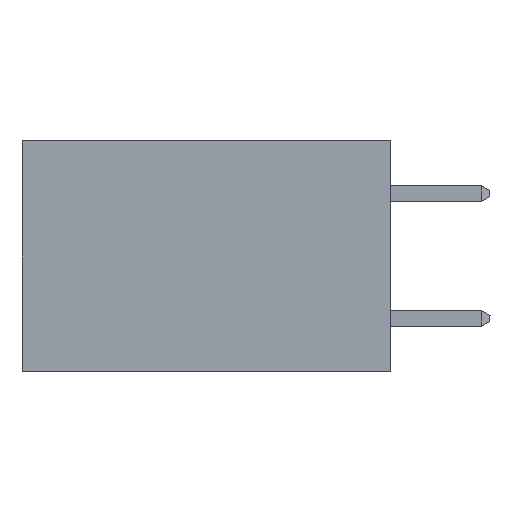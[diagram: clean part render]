
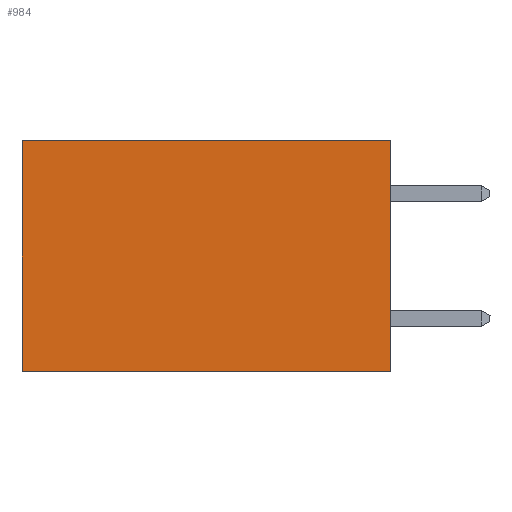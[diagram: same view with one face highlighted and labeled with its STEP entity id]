
A CAD part, left-side view. The second image highlights one B-rep face of the part: STEP entity #984.
In plain terms, the highlighted planar face has unit normal (-1, 0, 0).
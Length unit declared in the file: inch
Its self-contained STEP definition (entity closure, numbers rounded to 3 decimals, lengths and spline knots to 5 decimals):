
#61 = EDGE_CURVE ( 'NONE', #12855, #1841, #12094, .T. ) ;
#277 = DIRECTION ( 'NONE',  ( 0., 0., -1. ) ) ;
#730 = DIRECTION ( 'NONE',  ( 0., 1., 0. ) ) ;
#984 = ADVANCED_FACE ( 'NONE', ( #10764 ), #16046, .F. ) ;
#1525 = LINE ( 'NONE', #8451, #9704 ) ;
#1716 = ORIENTED_EDGE ( 'NONE', *, *, #5894, .F. ) ;
#1841 = VERTEX_POINT ( 'NONE', #11664 ) ;
#2413 = VECTOR ( 'NONE', #17200, 39.37008 ) ;
#2442 = DIRECTION ( 'NONE',  ( 1., 0., 0. ) ) ;
#2980 = ORIENTED_EDGE ( 'NONE', *, *, #6045, .F. ) ;
#4215 = CARTESIAN_POINT ( 'NONE',  ( 0.277, 0., 0. ) ) ;
#5894 = EDGE_CURVE ( 'NONE', #10501, #14128, #12106, .T. ) ;
#6045 = EDGE_CURVE ( 'NONE', #12855, #10501, #20850, .T. ) ;
#6291 = ORIENTED_EDGE ( 'NONE', *, *, #61, .T. ) ;
#6987 = EDGE_LOOP ( 'NONE', ( #19862, #1716, #2980, #6291 ) ) ;
#8206 = CARTESIAN_POINT ( 'NONE',  ( 0.277, 0., -0.37 ) ) ;
#8451 = CARTESIAN_POINT ( 'NONE',  ( 0.277, 0.59, -0.37 ) ) ;
#9471 = DIRECTION ( 'NONE',  ( 0., 0., -1. ) ) ;
#9704 = VECTOR ( 'NONE', #277, 39.37008 ) ;
#10501 = VERTEX_POINT ( 'NONE', #8206 ) ;
#10764 = FACE_OUTER_BOUND ( 'NONE', #6987, .T. ) ;
#11664 = CARTESIAN_POINT ( 'NONE',  ( 0.277, 0.59, 0. ) ) ;
#11853 = VECTOR ( 'NONE', #9471, 39.37008 ) ;
#12094 = LINE ( 'NONE', #4215, #20114 ) ;
#12106 = LINE ( 'NONE', #16774, #2413 ) ;
#12453 = CARTESIAN_POINT ( 'NONE',  ( 0.277, 0., -0.37 ) ) ;
#12855 = VERTEX_POINT ( 'NONE', #15340 ) ;
#14128 = VERTEX_POINT ( 'NONE', #15090 ) ;
#14478 = DIRECTION ( 'NONE',  ( 0., 0., -1. ) ) ;
#15012 = CARTESIAN_POINT ( 'NONE',  ( 0.277, 0., -0.37 ) ) ;
#15090 = CARTESIAN_POINT ( 'NONE',  ( 0.277, 0.59, -0.37 ) ) ;
#15340 = CARTESIAN_POINT ( 'NONE',  ( 0.277, 0., 0. ) ) ;
#16046 = PLANE ( 'NONE',  #18733 ) ;
#16774 = CARTESIAN_POINT ( 'NONE',  ( 0.277, 0., -0.37 ) ) ;
#16847 = EDGE_CURVE ( 'NONE', #1841, #14128, #1525, .T. ) ;
#17200 = DIRECTION ( 'NONE',  ( 0., 1., 0. ) ) ;
#18733 = AXIS2_PLACEMENT_3D ( 'NONE', #15012, #2442, #14478 ) ;
#19862 = ORIENTED_EDGE ( 'NONE', *, *, #16847, .T. ) ;
#20114 = VECTOR ( 'NONE', #730, 39.37008 ) ;
#20850 = LINE ( 'NONE', #12453, #11853 ) ;
